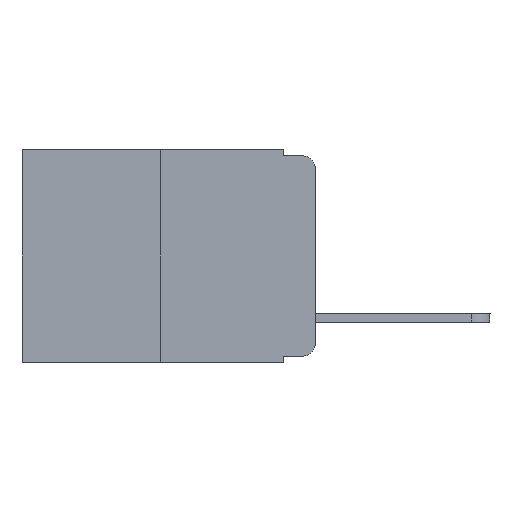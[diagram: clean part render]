
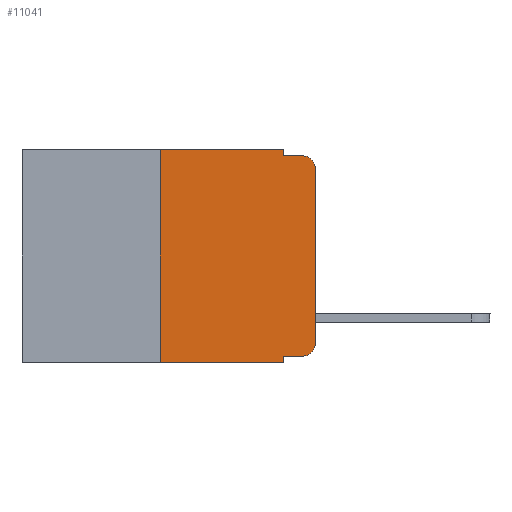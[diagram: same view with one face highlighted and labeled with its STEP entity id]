
A CAD part, left-side view. The second image highlights one B-rep face of the part: STEP entity #11041.
In plain terms, the highlighted planar face has unit normal (-1, 0, 0).
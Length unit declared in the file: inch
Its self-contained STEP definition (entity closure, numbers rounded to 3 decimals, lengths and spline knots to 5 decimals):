
#54 = EDGE_CURVE ( 'NONE', #2615, #11510, #9746, .T. ) ;
#1277 = DIRECTION ( 'NONE',  ( 1., 0., 0. ) ) ;
#1754 = VECTOR ( 'NONE', #6972, 39.37008 ) ;
#1898 = EDGE_CURVE ( 'NONE', #12253, #21137, #6425, .T. ) ;
#2211 = CARTESIAN_POINT ( 'NONE',  ( 0., 0.02, -0.313 ) ) ;
#2615 = VERTEX_POINT ( 'NONE', #2623 ) ;
#2623 = CARTESIAN_POINT ( 'NONE',  ( 0., 0.25, 0. ) ) ;
#2676 = VERTEX_POINT ( 'NONE', #15528 ) ;
#2916 = CARTESIAN_POINT ( 'NONE',  ( 0., 0.051, 0. ) ) ;
#3574 = EDGE_CURVE ( 'NONE', #2676, #2615, #20721, .T. ) ;
#3685 = DIRECTION ( 'NONE',  ( 0., 0., -1. ) ) ;
#3799 = DIRECTION ( 'NONE',  ( -1., 0., 0. ) ) ;
#4222 = LINE ( 'NONE', #7852, #10893 ) ;
#4676 = EDGE_LOOP ( 'NONE', ( #18020, #18304, #7181, #16954, #20916, #16424, #21671, #20076, #13650, #19394 ) ) ;
#4771 = EDGE_CURVE ( 'NONE', #11008, #10688, #7990, .T. ) ;
#4960 = VERTEX_POINT ( 'NONE', #16157 ) ;
#5141 = LINE ( 'NONE', #11842, #9811 ) ;
#5325 = AXIS2_PLACEMENT_3D ( 'NONE', #18869, #1277, #8101 ) ;
#5607 = CARTESIAN_POINT ( 'NONE',  ( 0., 0.051, -0.01 ) ) ;
#6381 = VECTOR ( 'NONE', #8054, 39.37008 ) ;
#6382 = FACE_OUTER_BOUND ( 'NONE', #4676, .T. ) ;
#6425 = CIRCLE ( 'NONE', #22413, 0.02 ) ;
#6741 = EDGE_CURVE ( 'NONE', #4960, #11008, #4222, .T. ) ;
#6972 = DIRECTION ( 'NONE',  ( 0., -1., 0. ) ) ;
#7181 = ORIENTED_EDGE ( 'NONE', *, *, #10782, .F. ) ;
#7852 = CARTESIAN_POINT ( 'NONE',  ( 0., 0.051, -0.333 ) ) ;
#7961 = DIRECTION ( 'NONE',  ( 0., -1., 0. ) ) ;
#7990 = CIRCLE ( 'NONE', #9429, 0.02 ) ;
#8054 = DIRECTION ( 'NONE',  ( 0., -1., 0. ) ) ;
#8101 = DIRECTION ( 'NONE',  ( 0., 0., -1. ) ) ;
#8586 = EDGE_CURVE ( 'NONE', #10688, #12253, #12122, .T. ) ;
#9429 = AXIS2_PLACEMENT_3D ( 'NONE', #2211, #3799, #3685 ) ;
#9571 = CARTESIAN_POINT ( 'NONE',  ( 0., 0.02, -0.333 ) ) ;
#9746 = LINE ( 'NONE', #16674, #6381 ) ;
#9792 = PLANE ( 'NONE',  #5325 ) ;
#9811 = VECTOR ( 'NONE', #10459, 39.37008 ) ;
#10177 = CARTESIAN_POINT ( 'NONE',  ( 0., 0.02, -0.03 ) ) ;
#10459 = DIRECTION ( 'NONE',  ( 0., 0., -1. ) ) ;
#10483 = CARTESIAN_POINT ( 'NONE',  ( 0., 0.473, -0.343 ) ) ;
#10688 = VERTEX_POINT ( 'NONE', #19002 ) ;
#10782 = EDGE_CURVE ( 'NONE', #19682, #21137, #12635, .T. ) ;
#10893 = VECTOR ( 'NONE', #7961, 39.37008 ) ;
#11008 = VERTEX_POINT ( 'NONE', #9571 ) ;
#11041 = ADVANCED_FACE ( 'NONE', ( #6382 ), #9792, .F. ) ;
#11510 = VERTEX_POINT ( 'NONE', #2916 ) ;
#11842 = CARTESIAN_POINT ( 'NONE',  ( 0., 0.051, 0. ) ) ;
#12084 = DIRECTION ( 'NONE',  ( 0., 0., 1. ) ) ;
#12122 = LINE ( 'NONE', #15636, #17460 ) ;
#12253 = VERTEX_POINT ( 'NONE', #17726 ) ;
#12487 = VERTEX_POINT ( 'NONE', #20338 ) ;
#12635 = LINE ( 'NONE', #5607, #13984 ) ;
#13235 = DIRECTION ( 'NONE',  ( 0., 0., -1. ) ) ;
#13367 = VECTOR ( 'NONE', #12084, 39.37008 ) ;
#13650 = ORIENTED_EDGE ( 'NONE', *, *, #6741, .T. ) ;
#13984 = VECTOR ( 'NONE', #19574, 39.37008 ) ;
#14499 = LINE ( 'NONE', #21456, #21490 ) ;
#15528 = CARTESIAN_POINT ( 'NONE',  ( 0., 0.25, -0.343 ) ) ;
#15594 = LINE ( 'NONE', #10483, #1754 ) ;
#15636 = CARTESIAN_POINT ( 'NONE',  ( 0., 0., 0. ) ) ;
#16157 = CARTESIAN_POINT ( 'NONE',  ( 0., 0.051, -0.333 ) ) ;
#16416 = CARTESIAN_POINT ( 'NONE',  ( 0., 0.051, -0.01 ) ) ;
#16424 = ORIENTED_EDGE ( 'NONE', *, *, #3574, .F. ) ;
#16607 = EDGE_CURVE ( 'NONE', #2676, #12487, #15594, .T. ) ;
#16674 = CARTESIAN_POINT ( 'NONE',  ( 0., 0.473, 0. ) ) ;
#16954 = ORIENTED_EDGE ( 'NONE', *, *, #18378, .F. ) ;
#17295 = CARTESIAN_POINT ( 'NONE',  ( 0., 0.25, 0. ) ) ;
#17460 = VECTOR ( 'NONE', #20430, 39.37008 ) ;
#17726 = CARTESIAN_POINT ( 'NONE',  ( 0., 0., -0.03 ) ) ;
#18020 = ORIENTED_EDGE ( 'NONE', *, *, #8586, .T. ) ;
#18265 = DIRECTION ( 'NONE',  ( 0., 0., -1. ) ) ;
#18304 = ORIENTED_EDGE ( 'NONE', *, *, #1898, .T. ) ;
#18378 = EDGE_CURVE ( 'NONE', #11510, #19682, #5141, .T. ) ;
#18690 = DIRECTION ( 'NONE',  ( -1., 0., 0. ) ) ;
#18869 = CARTESIAN_POINT ( 'NONE',  ( 0., 0.473, 0. ) ) ;
#19002 = CARTESIAN_POINT ( 'NONE',  ( 0., 0., -0.313 ) ) ;
#19121 = CARTESIAN_POINT ( 'NONE',  ( 0., 0.02, -0.01 ) ) ;
#19394 = ORIENTED_EDGE ( 'NONE', *, *, #4771, .T. ) ;
#19574 = DIRECTION ( 'NONE',  ( 0., -1., 0. ) ) ;
#19682 = VERTEX_POINT ( 'NONE', #16416 ) ;
#20076 = ORIENTED_EDGE ( 'NONE', *, *, #22134, .F. ) ;
#20338 = CARTESIAN_POINT ( 'NONE',  ( 0., 0.051, -0.343 ) ) ;
#20430 = DIRECTION ( 'NONE',  ( 0., 0., 1. ) ) ;
#20721 = LINE ( 'NONE', #17295, #13367 ) ;
#20916 = ORIENTED_EDGE ( 'NONE', *, *, #54, .F. ) ;
#21137 = VERTEX_POINT ( 'NONE', #19121 ) ;
#21456 = CARTESIAN_POINT ( 'NONE',  ( 0., 0.051, 0. ) ) ;
#21490 = VECTOR ( 'NONE', #18265, 39.37008 ) ;
#21671 = ORIENTED_EDGE ( 'NONE', *, *, #16607, .T. ) ;
#22134 = EDGE_CURVE ( 'NONE', #4960, #12487, #14499, .T. ) ;
#22413 = AXIS2_PLACEMENT_3D ( 'NONE', #10177, #18690, #13235 ) ;
